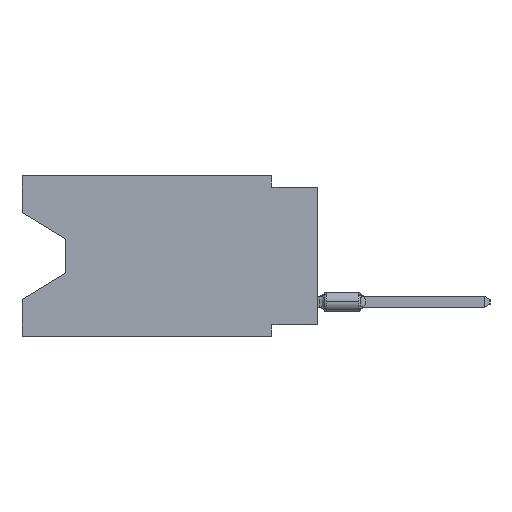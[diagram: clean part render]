
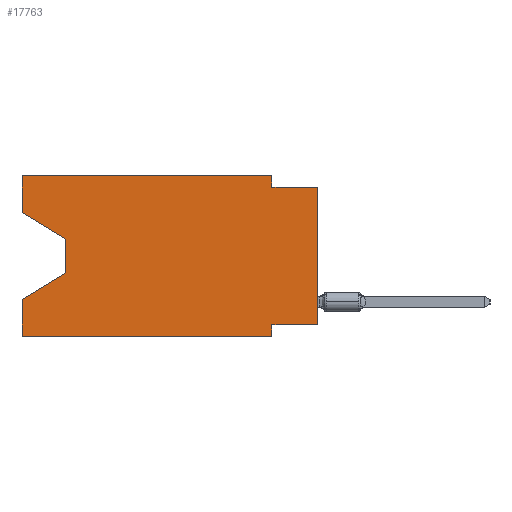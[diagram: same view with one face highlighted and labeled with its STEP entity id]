
A CAD part, left-side view. The second image highlights one B-rep face of the part: STEP entity #17763.
In plain terms, the highlighted planar face has unit normal (-1, 0, 0).
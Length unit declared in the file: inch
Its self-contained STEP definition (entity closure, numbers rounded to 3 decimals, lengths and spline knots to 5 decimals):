
#2656 = CARTESIAN_POINT ( 'NONE',  ( 0., 0.1, -0.35 ) ) ;
#2675 = EDGE_CURVE ( 'NONE', #4494, #40368, #49759, .T. ) ;
#4494 = VERTEX_POINT ( 'NONE', #47831 ) ;
#4942 = VERTEX_POINT ( 'NONE', #9982 ) ;
#5105 = ORIENTED_EDGE ( 'NONE', *, *, #48069, .T. ) ;
#5113 = CARTESIAN_POINT ( 'NONE',  ( 0., 0.55, -0.138 ) ) ;
#5213 = ORIENTED_EDGE ( 'NONE', *, *, #44451, .F. ) ;
#5738 = CARTESIAN_POINT ( 'NONE',  ( 0., 0.1, -0.325 ) ) ;
#5789 = ORIENTED_EDGE ( 'NONE', *, *, #13527, .T. ) ;
#7715 = LINE ( 'NONE', #37317, #50607 ) ;
#8818 = ORIENTED_EDGE ( 'NONE', *, *, #11506, .T. ) ;
#9005 = CARTESIAN_POINT ( 'NONE',  ( 0., 0.645, -0.26975 ) ) ;
#9358 = DIRECTION ( 'NONE',  ( 0., 0., 1. ) ) ;
#9598 = VERTEX_POINT ( 'NONE', #21650 ) ;
#9698 = VECTOR ( 'NONE', #21437, 39.37008 ) ;
#9982 = CARTESIAN_POINT ( 'NONE',  ( 0., 0.645, -0.35 ) ) ;
#10112 = EDGE_CURVE ( 'NONE', #4494, #53150, #29737, .T. ) ;
#10879 = DIRECTION ( 'NONE',  ( 0., 0., -1. ) ) ;
#11482 = ORIENTED_EDGE ( 'NONE', *, *, #37553, .F. ) ;
#11506 = EDGE_CURVE ( 'NONE', #40368, #24784, #51032, .T. ) ;
#12019 = LINE ( 'NONE', #16103, #41923 ) ;
#12522 = CARTESIAN_POINT ( 'NONE',  ( 0., 0.645, -0.08025 ) ) ;
#13468 = CARTESIAN_POINT ( 'NONE',  ( 0., 0.55, -0.212 ) ) ;
#13527 = EDGE_CURVE ( 'NONE', #24784, #49544, #50973, .T. ) ;
#13730 = DIRECTION ( 'NONE',  ( 0., 0.855, -0.519 ) ) ;
#14448 = EDGE_CURVE ( 'NONE', #53150, #20190, #18487, .T. ) ;
#14481 = CARTESIAN_POINT ( 'NONE',  ( 0., 0.645, 0. ) ) ;
#16103 = CARTESIAN_POINT ( 'NONE',  ( 0., 0., -0.025 ) ) ;
#16950 = CARTESIAN_POINT ( 'NONE',  ( 0., 0.55, -0.212 ) ) ;
#17630 = VERTEX_POINT ( 'NONE', #5738 ) ;
#17654 = CARTESIAN_POINT ( 'NONE',  ( 0., 0., -0.325 ) ) ;
#17716 = VECTOR ( 'NONE', #13730, 39.37008 ) ;
#17763 = ADVANCED_FACE ( 'NONE', ( #17948 ), #34521, .F. ) ;
#17916 = CARTESIAN_POINT ( 'NONE',  ( 0., 0.1, 0. ) ) ;
#17948 = FACE_OUTER_BOUND ( 'NONE', #28036, .T. ) ;
#18487 = LINE ( 'NONE', #35876, #49817 ) ;
#19042 = VECTOR ( 'NONE', #51300, 39.37008 ) ;
#19421 = LINE ( 'NONE', #36004, #19042 ) ;
#20190 = VERTEX_POINT ( 'NONE', #17916 ) ;
#21437 = DIRECTION ( 'NONE',  ( 0., 0., 1. ) ) ;
#21650 = CARTESIAN_POINT ( 'NONE',  ( 0., 0., -0.025 ) ) ;
#21978 = LINE ( 'NONE', #51061, #9698 ) ;
#23378 = DIRECTION ( 'NONE',  ( 0., -1., 0. ) ) ;
#23526 = ORIENTED_EDGE ( 'NONE', *, *, #27055, .T. ) ;
#24217 = DIRECTION ( 'NONE',  ( 0., 0., -1. ) ) ;
#24377 = AXIS2_PLACEMENT_3D ( 'NONE', #35611, #31803, #10879 ) ;
#24488 = ORIENTED_EDGE ( 'NONE', *, *, #2675, .T. ) ;
#24784 = VERTEX_POINT ( 'NONE', #16950 ) ;
#24893 = ORIENTED_EDGE ( 'NONE', *, *, #42322, .F. ) ;
#25588 = ORIENTED_EDGE ( 'NONE', *, *, #14448, .F. ) ;
#27055 = EDGE_CURVE ( 'NONE', #4942, #31271, #7715, .T. ) ;
#28036 = EDGE_LOOP ( 'NONE', ( #24488, #8818, #5789, #38596, #23526, #52578, #11482, #5105, #24893, #5213, #25588, #41968 ) ) ;
#29092 = DIRECTION ( 'NONE',  ( 0., -0.855, -0.519 ) ) ;
#29737 = LINE ( 'NONE', #30013, #35455 ) ;
#30013 = CARTESIAN_POINT ( 'NONE',  ( 0., 0.645, 0. ) ) ;
#31271 = VERTEX_POINT ( 'NONE', #2656 ) ;
#31413 = VECTOR ( 'NONE', #24217, 39.37008 ) ;
#31803 = DIRECTION ( 'NONE',  ( 1., 0., 0. ) ) ;
#31854 = CARTESIAN_POINT ( 'NONE',  ( 0., 0.1, -0.35 ) ) ;
#32588 = LINE ( 'NONE', #44835, #39856 ) ;
#34047 = EDGE_CURVE ( 'NONE', #4942, #49544, #21978, .T. ) ;
#34521 = PLANE ( 'NONE',  #24377 ) ;
#35151 = DIRECTION ( 'NONE',  ( 0., 0., -1. ) ) ;
#35160 = VECTOR ( 'NONE', #29092, 39.37008 ) ;
#35455 = VECTOR ( 'NONE', #9358, 39.37008 ) ;
#35611 = CARTESIAN_POINT ( 'NONE',  ( 0., 0.645, 0. ) ) ;
#35876 = CARTESIAN_POINT ( 'NONE',  ( 0., 0.645, 0. ) ) ;
#36004 = CARTESIAN_POINT ( 'NONE',  ( 0., 0., -0.325 ) ) ;
#36208 = LINE ( 'NONE', #31854, #31413 ) ;
#37317 = CARTESIAN_POINT ( 'NONE',  ( 0., 0.645, -0.35 ) ) ;
#37553 = EDGE_CURVE ( 'NONE', #38901, #17630, #19421, .T. ) ;
#37702 = CARTESIAN_POINT ( 'NONE',  ( 0., 0.1, -0.025 ) ) ;
#38366 = VECTOR ( 'NONE', #42341, 39.37008 ) ;
#38596 = ORIENTED_EDGE ( 'NONE', *, *, #34047, .F. ) ;
#38901 = VERTEX_POINT ( 'NONE', #17654 ) ;
#39231 = CARTESIAN_POINT ( 'NONE',  ( 0., 0.1, 0. ) ) ;
#39856 = VECTOR ( 'NONE', #40507, 39.37008 ) ;
#40368 = VERTEX_POINT ( 'NONE', #41726 ) ;
#40507 = DIRECTION ( 'NONE',  ( 0., 0., 1. ) ) ;
#41151 = DIRECTION ( 'NONE',  ( 0., -1., 0. ) ) ;
#41650 = DIRECTION ( 'NONE',  ( 0., -1., 0. ) ) ;
#41726 = CARTESIAN_POINT ( 'NONE',  ( 0., 0.55, -0.138 ) ) ;
#41838 = VERTEX_POINT ( 'NONE', #37702 ) ;
#41923 = VECTOR ( 'NONE', #41650, 39.37008 ) ;
#41968 = ORIENTED_EDGE ( 'NONE', *, *, #10112, .F. ) ;
#42322 = EDGE_CURVE ( 'NONE', #41838, #9598, #12019, .T. ) ;
#42341 = DIRECTION ( 'NONE',  ( 0., 0., -1. ) ) ;
#44451 = EDGE_CURVE ( 'NONE', #20190, #41838, #52264, .T. ) ;
#44835 = CARTESIAN_POINT ( 'NONE',  ( 0., 0., 0. ) ) ;
#47831 = CARTESIAN_POINT ( 'NONE',  ( 0., 0.645, -0.08025 ) ) ;
#48069 = EDGE_CURVE ( 'NONE', #38901, #9598, #32588, .T. ) ;
#49544 = VERTEX_POINT ( 'NONE', #9005 ) ;
#49759 = LINE ( 'NONE', #12522, #35160 ) ;
#49817 = VECTOR ( 'NONE', #23378, 39.37008 ) ;
#50607 = VECTOR ( 'NONE', #41151, 39.37008 ) ;
#50973 = LINE ( 'NONE', #13468, #17716 ) ;
#51032 = LINE ( 'NONE', #5113, #38366 ) ;
#51061 = CARTESIAN_POINT ( 'NONE',  ( 0., 0.645, 0. ) ) ;
#51300 = DIRECTION ( 'NONE',  ( 0., 1., 0. ) ) ;
#51638 = VECTOR ( 'NONE', #35151, 39.37008 ) ;
#52264 = LINE ( 'NONE', #39231, #51638 ) ;
#52578 = ORIENTED_EDGE ( 'NONE', *, *, #53256, .F. ) ;
#53150 = VERTEX_POINT ( 'NONE', #14481 ) ;
#53256 = EDGE_CURVE ( 'NONE', #17630, #31271, #36208, .T. ) ;
